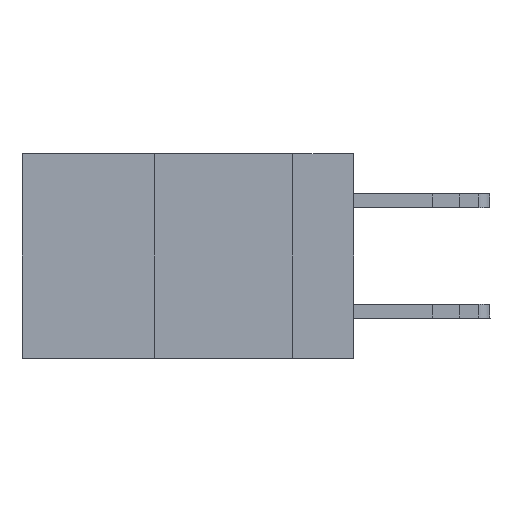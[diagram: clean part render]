
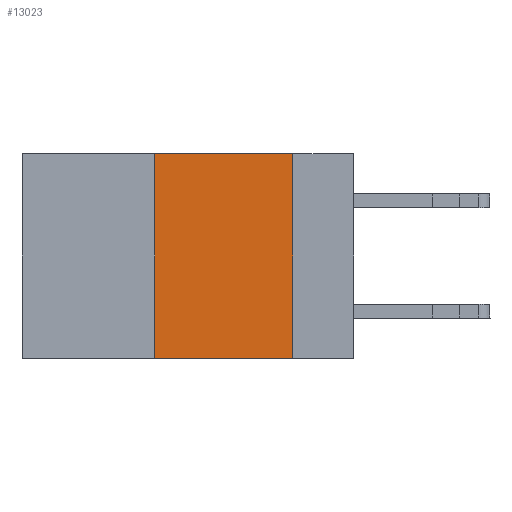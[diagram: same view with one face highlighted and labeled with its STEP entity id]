
A CAD part, left-side view. The second image highlights one B-rep face of the part: STEP entity #13023.
In plain terms, the highlighted planar face has unit normal (-1, 0, 0).
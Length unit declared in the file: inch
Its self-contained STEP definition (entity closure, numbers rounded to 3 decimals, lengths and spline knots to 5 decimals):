
#1468 = ORIENTED_EDGE ( 'NONE', *, *, #15561, .T. ) ;
#2271 = DIRECTION ( 'NONE',  ( 1., 0., 0. ) ) ;
#5964 = EDGE_LOOP ( 'NONE', ( #12310, #6785, #10879, #1468 ) ) ;
#6497 = VERTEX_POINT ( 'NONE', #14959 ) ;
#6685 = FACE_OUTER_BOUND ( 'NONE', #5964, .T. ) ;
#6785 = ORIENTED_EDGE ( 'NONE', *, *, #7157, .F. ) ;
#6987 = VERTEX_POINT ( 'NONE', #18380 ) ;
#7157 = EDGE_CURVE ( 'NONE', #21791, #6497, #9242, .T. ) ;
#7231 = CARTESIAN_POINT ( 'NONE',  ( 0., 0.11, 0. ) ) ;
#7624 = DIRECTION ( 'NONE',  ( 0., -1., 0. ) ) ;
#7894 = CARTESIAN_POINT ( 'NONE',  ( 0., 0.36, 0. ) ) ;
#7990 = DIRECTION ( 'NONE',  ( 0., 0., 1. ) ) ;
#8420 = CARTESIAN_POINT ( 'NONE',  ( 0., 0.36, 0. ) ) ;
#9242 = LINE ( 'NONE', #27478, #21045 ) ;
#9472 = LINE ( 'NONE', #7894, #24986 ) ;
#9502 = DIRECTION ( 'NONE',  ( 0., 0., -1. ) ) ;
#10827 = EDGE_CURVE ( 'NONE', #6497, #6987, #23875, .T. ) ;
#10879 = ORIENTED_EDGE ( 'NONE', *, *, #18919, .F. ) ;
#11186 = CARTESIAN_POINT ( 'NONE',  ( 0., 0.6, 0. ) ) ;
#12063 = VECTOR ( 'NONE', #7624, 39.37008 ) ;
#12310 = ORIENTED_EDGE ( 'NONE', *, *, #10827, .F. ) ;
#13023 = ADVANCED_FACE ( 'NONE', ( #6685 ), #20113, .F. ) ;
#14466 = DIRECTION ( 'NONE',  ( 0., -1., 0. ) ) ;
#14959 = CARTESIAN_POINT ( 'NONE',  ( 0., 0.11, 0. ) ) ;
#15561 = EDGE_CURVE ( 'NONE', #15888, #6987, #16542, .T. ) ;
#15888 = VERTEX_POINT ( 'NONE', #21702 ) ;
#16405 = CARTESIAN_POINT ( 'NONE',  ( 0., 0.6, -0.37 ) ) ;
#16542 = LINE ( 'NONE', #16405, #12063 ) ;
#17416 = AXIS2_PLACEMENT_3D ( 'NONE', #11186, #2271, #20208 ) ;
#18380 = CARTESIAN_POINT ( 'NONE',  ( 0., 0.11, -0.37 ) ) ;
#18919 = EDGE_CURVE ( 'NONE', #15888, #21791, #9472, .T. ) ;
#20113 = PLANE ( 'NONE',  #17416 ) ;
#20208 = DIRECTION ( 'NONE',  ( 0., 0., -1. ) ) ;
#21045 = VECTOR ( 'NONE', #14466, 39.37008 ) ;
#21702 = CARTESIAN_POINT ( 'NONE',  ( 0., 0.36, -0.37 ) ) ;
#21791 = VERTEX_POINT ( 'NONE', #8420 ) ;
#23513 = VECTOR ( 'NONE', #9502, 39.37008 ) ;
#23875 = LINE ( 'NONE', #7231, #23513 ) ;
#24986 = VECTOR ( 'NONE', #7990, 39.37008 ) ;
#27478 = CARTESIAN_POINT ( 'NONE',  ( 0., 0.6, 0. ) ) ;
